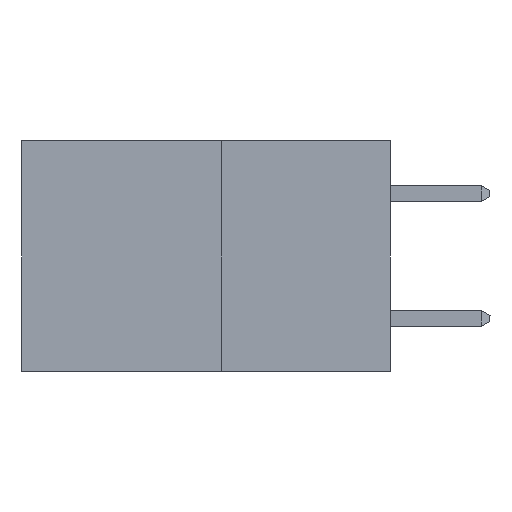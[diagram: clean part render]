
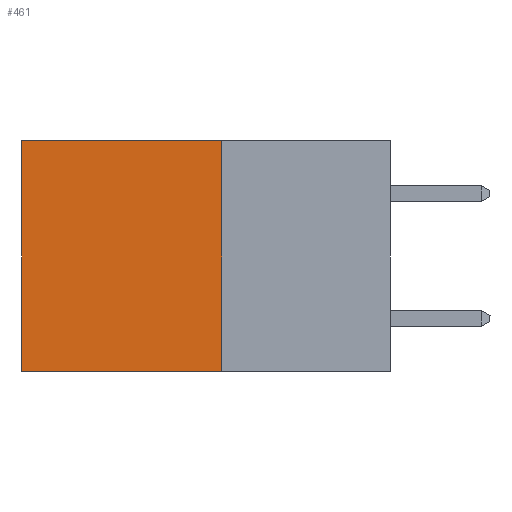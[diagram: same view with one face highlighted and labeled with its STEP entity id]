
A CAD part, left-side view. The second image highlights one B-rep face of the part: STEP entity #461.
In plain terms, the highlighted planar face has unit normal (-1, 0, 0).
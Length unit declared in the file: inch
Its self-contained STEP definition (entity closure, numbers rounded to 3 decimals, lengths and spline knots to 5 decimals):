
#271 = ORIENTED_EDGE ( 'NONE', *, *, #22103, .T. ) ;
#461 = ADVANCED_FACE ( 'NONE', ( #4574 ), #9437, .F. ) ;
#491 = VERTEX_POINT ( 'NONE', #10066 ) ;
#566 = ORIENTED_EDGE ( 'NONE', *, *, #17843, .F. ) ;
#614 = DIRECTION ( 'NONE',  ( 0., 0., -1. ) ) ;
#1883 = EDGE_CURVE ( 'NONE', #22886, #9080, #10802, .T. ) ;
#2813 = VECTOR ( 'NONE', #12646, 39.37008 ) ;
#4574 = FACE_OUTER_BOUND ( 'NONE', #10451, .T. ) ;
#5367 = CARTESIAN_POINT ( 'NONE',  ( 0.277, 0.27, -0.37 ) ) ;
#7009 = DIRECTION ( 'NONE',  ( 1., 0., 0. ) ) ;
#8451 = CARTESIAN_POINT ( 'NONE',  ( 0.277, 0.27, 0. ) ) ;
#9009 = VECTOR ( 'NONE', #22558, 39.37008 ) ;
#9080 = VERTEX_POINT ( 'NONE', #5367 ) ;
#9437 = PLANE ( 'NONE',  #20260 ) ;
#9566 = LINE ( 'NONE', #20793, #9009 ) ;
#9672 = DIRECTION ( 'NONE',  ( 0., 0., -1. ) ) ;
#9766 = LINE ( 'NONE', #20484, #18719 ) ;
#10066 = CARTESIAN_POINT ( 'NONE',  ( 0.277, 0.59, -0.37 ) ) ;
#10451 = EDGE_LOOP ( 'NONE', ( #13707, #566, #11058, #271 ) ) ;
#10796 = CARTESIAN_POINT ( 'NONE',  ( 0.277, 0.27, -0.37 ) ) ;
#10802 = LINE ( 'NONE', #12337, #19735 ) ;
#11058 = ORIENTED_EDGE ( 'NONE', *, *, #1883, .F. ) ;
#12337 = CARTESIAN_POINT ( 'NONE',  ( 0.277, 0.27, -0.37 ) ) ;
#12646 = DIRECTION ( 'NONE',  ( 0., 1., 0. ) ) ;
#13656 = LINE ( 'NONE', #10796, #2813 ) ;
#13707 = ORIENTED_EDGE ( 'NONE', *, *, #15487, .T. ) ;
#13826 = CARTESIAN_POINT ( 'NONE',  ( 0.277, 0.59, 0. ) ) ;
#15487 = EDGE_CURVE ( 'NONE', #20871, #491, #9766, .T. ) ;
#17843 = EDGE_CURVE ( 'NONE', #9080, #491, #13656, .T. ) ;
#18595 = CARTESIAN_POINT ( 'NONE',  ( 0.277, 0.27, -0.37 ) ) ;
#18719 = VECTOR ( 'NONE', #614, 39.37008 ) ;
#19735 = VECTOR ( 'NONE', #9672, 39.37008 ) ;
#20260 = AXIS2_PLACEMENT_3D ( 'NONE', #18595, #7009, #20353 ) ;
#20353 = DIRECTION ( 'NONE',  ( 0., 0., -1. ) ) ;
#20484 = CARTESIAN_POINT ( 'NONE',  ( 0.277, 0.59, -0.37 ) ) ;
#20793 = CARTESIAN_POINT ( 'NONE',  ( 0.277, 0.27, 0. ) ) ;
#20871 = VERTEX_POINT ( 'NONE', #13826 ) ;
#22103 = EDGE_CURVE ( 'NONE', #22886, #20871, #9566, .T. ) ;
#22558 = DIRECTION ( 'NONE',  ( 0., 1., 0. ) ) ;
#22886 = VERTEX_POINT ( 'NONE', #8451 ) ;
